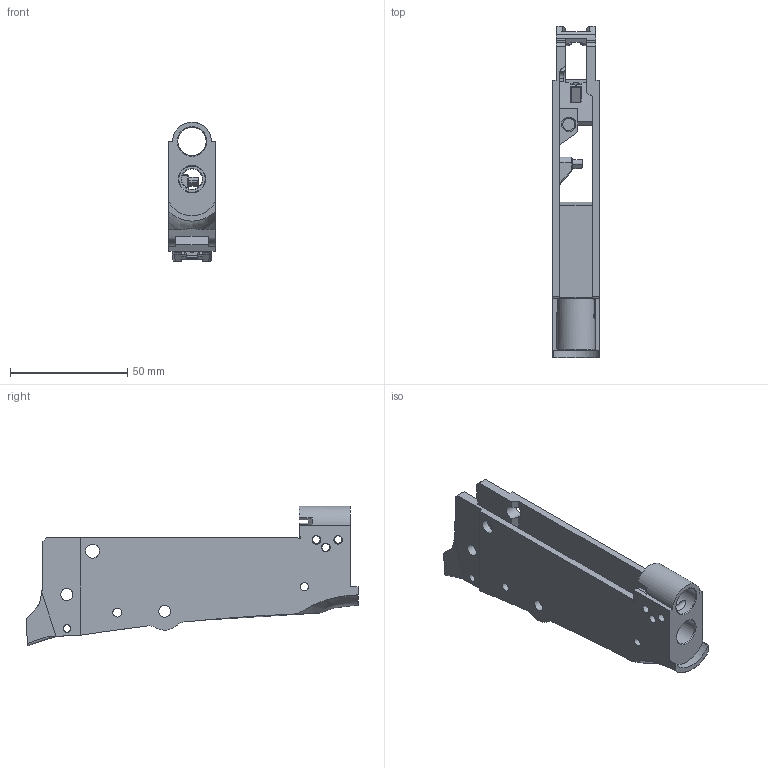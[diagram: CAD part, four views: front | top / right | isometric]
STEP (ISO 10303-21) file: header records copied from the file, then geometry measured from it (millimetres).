
FILE_DESCRIPTION(/* description */ (''),/* implementation_level */ '2;1');
FILE_NAME(/* name */ 'P.L.A. Frame with lever bump.step',/* time_stamp */ '2022-06-19T00:28:49-05:00',/* author */ (''),/* organization */ (''),/* preprocessor_version */ 'ST-DEVELOPER v19',/* originating_system */ 'Autodesk Translation Framework v11.7.0.108',/* authorisation */ '');
FILE_SCHEMA (('AUTOMOTIVE_DESIGN { 1 0 10303 214 3 1 1 }'));
Length unit declared in the file: millimetre
Products named in the file (1): P.L.A. Frame Lever Bump
Bounding box: 20 x 141.88 x 59.66 mm (x, y, z)
Volume: 42736.5 mm3; surface area: 27125.8 mm2
Topology: 1 solids, 1 shells, 203 faces, 584 edges, 382 vertices
Faces by surface type: plane 123, cylinder 56, cone 15, bspline 9
Full cylindrical faces by diameter (mm): 3.2 x3, 3.5 x1, 3.61 x2, 3.8 x2, 4.2 x1, 5 x1, 5.2 x4, 6 x2, 8.7 x1, 11.2 x1, 12.1 x1
Entity records: 7451 total; most frequent: CARTESIAN_POINT 1923, ORIENTED_EDGE 1168, DIRECTION 1125, EDGE_CURVE 584, LINE 389, VECTOR 389, VERTEX_POINT 382, AXIS2_PLACEMENT_3D 368
